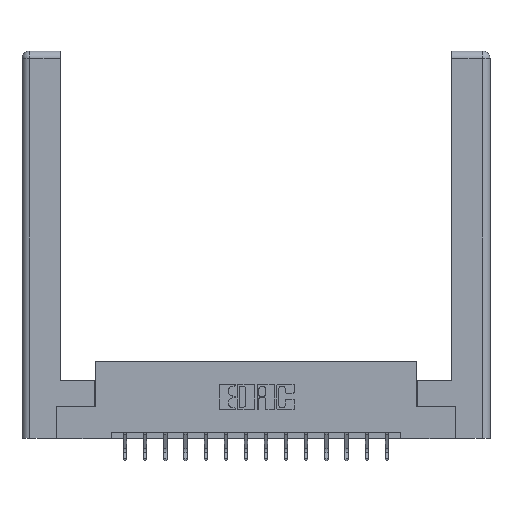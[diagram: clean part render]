
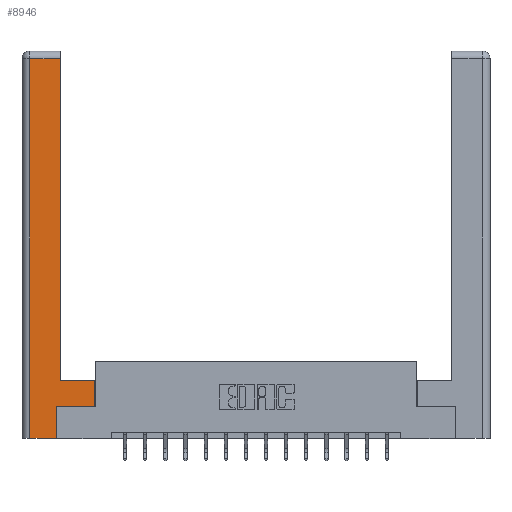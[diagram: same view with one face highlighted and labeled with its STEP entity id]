
A CAD part, top view. The second image highlights one B-rep face of the part: STEP entity #8946.
In plain terms, the highlighted planar face has unit normal (0, 0, 1).
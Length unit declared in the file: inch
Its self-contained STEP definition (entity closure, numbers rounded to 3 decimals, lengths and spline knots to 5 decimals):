
#41 = CARTESIAN_POINT ( 'NONE',  ( 0.0615, 0., 0. ) ) ;
#166 = CARTESIAN_POINT ( 'NONE',  ( 0.295, 2.94, 0. ) ) ;
#270 = VERTEX_POINT ( 'NONE', #1914 ) ;
#302 = DIRECTION ( 'NONE',  ( 0., 1., 0. ) ) ;
#675 = EDGE_CURVE ( 'NONE', #3605, #14730, #6348, .T. ) ;
#685 = CARTESIAN_POINT ( 'NONE',  ( 0.295, 0.45, 0. ) ) ;
#850 = ORIENTED_EDGE ( 'NONE', *, *, #675, .T. ) ;
#1609 = CARTESIAN_POINT ( 'NONE',  ( 0.565, 0.45, 0. ) ) ;
#1686 = CARTESIAN_POINT ( 'NONE',  ( 0.265, 0., 0. ) ) ;
#1913 = ORIENTED_EDGE ( 'NONE', *, *, #3994, .T. ) ;
#1914 = CARTESIAN_POINT ( 'NONE',  ( 0.0615, 0., 0. ) ) ;
#2382 = VECTOR ( 'NONE', #14515, 39.37008 ) ;
#2733 = ORIENTED_EDGE ( 'NONE', *, *, #8380, .T. ) ;
#3109 = CARTESIAN_POINT ( 'NONE',  ( 0.265, 0.245, 0. ) ) ;
#3174 = VERTEX_POINT ( 'NONE', #7258 ) ;
#3380 = CARTESIAN_POINT ( 'NONE',  ( 0., 0., 0. ) ) ;
#3605 = VERTEX_POINT ( 'NONE', #7312 ) ;
#3748 = CARTESIAN_POINT ( 'NONE',  ( 0.565, 0.245, 0. ) ) ;
#3861 = VECTOR ( 'NONE', #15240, 39.37008 ) ;
#3912 = EDGE_LOOP ( 'NONE', ( #1913, #2733, #15523, #10431, #10027, #7924, #850, #12417 ) ) ;
#3994 = EDGE_CURVE ( 'NONE', #8985, #16332, #13901, .T. ) ;
#4548 = VECTOR ( 'NONE', #8654, 39.37008 ) ;
#4698 = VECTOR ( 'NONE', #302, 39.37008 ) ;
#5298 = LINE ( 'NONE', #12077, #10990 ) ;
#5369 = LINE ( 'NONE', #9868, #4548 ) ;
#5655 = VECTOR ( 'NONE', #8925, 39.37008 ) ;
#5711 = VECTOR ( 'NONE', #16861, 39.37008 ) ;
#5904 = EDGE_CURVE ( 'NONE', #14730, #8985, #5369, .T. ) ;
#5944 = VERTEX_POINT ( 'NONE', #6001 ) ;
#6001 = CARTESIAN_POINT ( 'NONE',  ( 0.265, 0.245, 0. ) ) ;
#6348 = LINE ( 'NONE', #1609, #4698 ) ;
#7258 = CARTESIAN_POINT ( 'NONE',  ( 0.0615, 2.94, 0. ) ) ;
#7312 = CARTESIAN_POINT ( 'NONE',  ( 0.565, 0.245, 0. ) ) ;
#7794 = FACE_OUTER_BOUND ( 'NONE', #3912, .T. ) ;
#7924 = ORIENTED_EDGE ( 'NONE', *, *, #8529, .T. ) ;
#7933 = EDGE_CURVE ( 'NONE', #3174, #270, #13369, .T. ) ;
#8229 = LINE ( 'NONE', #15756, #5711 ) ;
#8380 = EDGE_CURVE ( 'NONE', #16332, #3174, #8229, .T. ) ;
#8529 = EDGE_CURVE ( 'NONE', #5944, #3605, #14166, .T. ) ;
#8654 = DIRECTION ( 'NONE',  ( -1., 0., 0. ) ) ;
#8658 = EDGE_CURVE ( 'NONE', #270, #13615, #5298, .T. ) ;
#8783 = AXIS2_PLACEMENT_3D ( 'NONE', #3380, #13925, #15323 ) ;
#8925 = DIRECTION ( 'NONE',  ( 0., 1., 0. ) ) ;
#8946 = ADVANCED_FACE ( 'NONE', ( #7794 ), #12697, .F. ) ;
#8985 = VERTEX_POINT ( 'NONE', #685 ) ;
#9320 = VECTOR ( 'NONE', #16578, 39.37008 ) ;
#9868 = CARTESIAN_POINT ( 'NONE',  ( 0.295, 0.45, 0. ) ) ;
#10027 = ORIENTED_EDGE ( 'NONE', *, *, #14474, .T. ) ;
#10431 = ORIENTED_EDGE ( 'NONE', *, *, #8658, .T. ) ;
#10609 = LINE ( 'NONE', #3109, #3861 ) ;
#10990 = VECTOR ( 'NONE', #14688, 39.37008 ) ;
#11612 = CARTESIAN_POINT ( 'NONE',  ( 0.295, 3., 0. ) ) ;
#12077 = CARTESIAN_POINT ( 'NONE',  ( 0.265, 0., 0. ) ) ;
#12417 = ORIENTED_EDGE ( 'NONE', *, *, #5904, .T. ) ;
#12697 = PLANE ( 'NONE',  #8783 ) ;
#13369 = LINE ( 'NONE', #41, #9320 ) ;
#13615 = VERTEX_POINT ( 'NONE', #1686 ) ;
#13901 = LINE ( 'NONE', #11612, #5655 ) ;
#13925 = DIRECTION ( 'NONE',  ( 0., 0., -1. ) ) ;
#14166 = LINE ( 'NONE', #3748, #2382 ) ;
#14474 = EDGE_CURVE ( 'NONE', #13615, #5944, #10609, .T. ) ;
#14515 = DIRECTION ( 'NONE',  ( 1., 0., 0. ) ) ;
#14688 = DIRECTION ( 'NONE',  ( 1., 0., 0. ) ) ;
#14730 = VERTEX_POINT ( 'NONE', #16619 ) ;
#15240 = DIRECTION ( 'NONE',  ( 0., 1., 0. ) ) ;
#15323 = DIRECTION ( 'NONE',  ( -1., 0., 0. ) ) ;
#15523 = ORIENTED_EDGE ( 'NONE', *, *, #7933, .T. ) ;
#15756 = CARTESIAN_POINT ( 'NONE',  ( 0.0615, 2.94, 0. ) ) ;
#16332 = VERTEX_POINT ( 'NONE', #166 ) ;
#16578 = DIRECTION ( 'NONE',  ( 0., -1., 0. ) ) ;
#16619 = CARTESIAN_POINT ( 'NONE',  ( 0.565, 0.45, 0. ) ) ;
#16861 = DIRECTION ( 'NONE',  ( -1., 0., 0. ) ) ;
